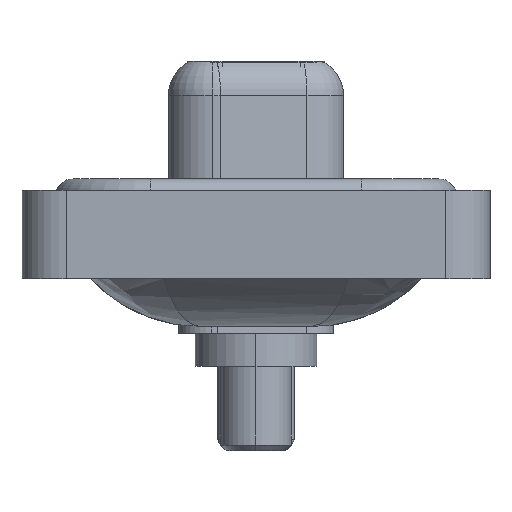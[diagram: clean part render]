
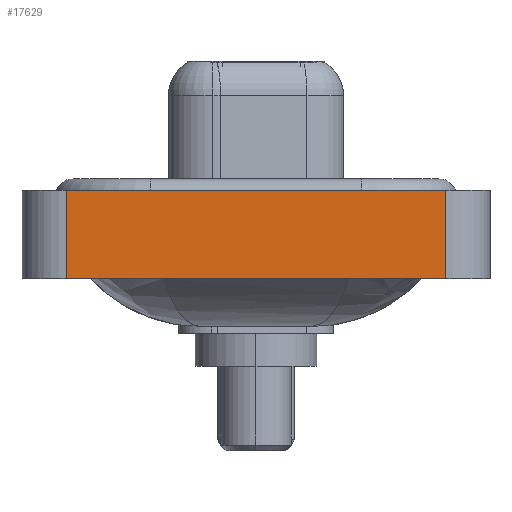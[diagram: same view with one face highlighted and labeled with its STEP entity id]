
A CAD part, left-side view. The second image highlights one B-rep face of the part: STEP entity #17629.
In plain terms, the highlighted planar face has unit normal (-1, 0, 0).
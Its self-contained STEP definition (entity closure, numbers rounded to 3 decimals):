
#199 = EDGE_CURVE ( 'NONE', #1530, #1700, #13760, .T. ) ;
#612 = VECTOR ( 'NONE', #1816, 1000. ) ;
#966 = EDGE_LOOP ( 'NONE', ( #10631, #2546, #10385, #10535 ) ) ;
#1051 = DIRECTION ( 'NONE',  ( 0., -1., 0. ) ) ;
#1530 = VERTEX_POINT ( 'NONE', #6923 ) ;
#1700 = VERTEX_POINT ( 'NONE', #15307 ) ;
#1816 = DIRECTION ( 'NONE',  ( 0., -1., 0. ) ) ;
#2057 = DIRECTION ( 'NONE',  ( 0., 0., 1. ) ) ;
#2225 = AXIS2_PLACEMENT_3D ( 'NONE', #12593, #20185, #7438 ) ;
#2546 = ORIENTED_EDGE ( 'NONE', *, *, #199, .F. ) ;
#2754 = CARTESIAN_POINT ( 'NONE',  ( -7.35, 8.55, -3.6 ) ) ;
#2757 = VERTEX_POINT ( 'NONE', #2754 ) ;
#3218 = VECTOR ( 'NONE', #2057, 1000. ) ;
#3789 = EDGE_CURVE ( 'NONE', #2757, #1530, #6277, .T. ) ;
#4487 = PLANE ( 'NONE',  #2225 ) ;
#6277 = LINE ( 'NONE', #10143, #3218 ) ;
#6923 = CARTESIAN_POINT ( 'NONE',  ( -7.35, 8.55, 0.4 ) ) ;
#7438 = DIRECTION ( 'NONE',  ( 0., 0., 1. ) ) ;
#9422 = EDGE_CURVE ( 'NONE', #14040, #1700, #11163, .T. ) ;
#9811 = CARTESIAN_POINT ( 'NONE',  ( -7.35, -8.55, -3.6 ) ) ;
#10143 = CARTESIAN_POINT ( 'NONE',  ( -7.35, 8.55, -3.6 ) ) ;
#10385 = ORIENTED_EDGE ( 'NONE', *, *, #3789, .F. ) ;
#10535 = ORIENTED_EDGE ( 'NONE', *, *, #10958, .T. ) ;
#10631 = ORIENTED_EDGE ( 'NONE', *, *, #9422, .T. ) ;
#10958 = EDGE_CURVE ( 'NONE', #2757, #14040, #14821, .T. ) ;
#11163 = LINE ( 'NONE', #17332, #13827 ) ;
#12593 = CARTESIAN_POINT ( 'NONE',  ( -7.35, -8.55, -3.6 ) ) ;
#12880 = VECTOR ( 'NONE', #1051, 1000. ) ;
#13165 = CARTESIAN_POINT ( 'NONE',  ( -7.35, -8.55, -3.6 ) ) ;
#13760 = LINE ( 'NONE', #17001, #12880 ) ;
#13827 = VECTOR ( 'NONE', #15875, 1000. ) ;
#13838 = FACE_OUTER_BOUND ( 'NONE', #966, .T. ) ;
#14040 = VERTEX_POINT ( 'NONE', #13165 ) ;
#14821 = LINE ( 'NONE', #9811, #612 ) ;
#15307 = CARTESIAN_POINT ( 'NONE',  ( -7.35, -8.55, 0.4 ) ) ;
#15875 = DIRECTION ( 'NONE',  ( 0., 0., 1. ) ) ;
#17001 = CARTESIAN_POINT ( 'NONE',  ( -7.35, -8.55, 0.4 ) ) ;
#17332 = CARTESIAN_POINT ( 'NONE',  ( -7.35, -8.55, -3.6 ) ) ;
#17629 = ADVANCED_FACE ( 'NONE', ( #13838 ), #4487, .T. ) ;
#20185 = DIRECTION ( 'NONE',  ( -1., 0., 0. ) ) ;
